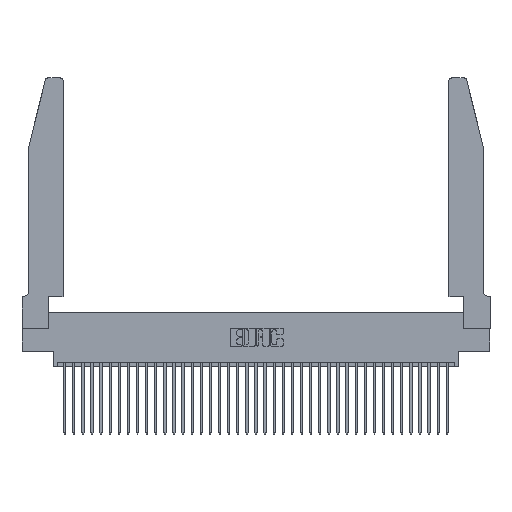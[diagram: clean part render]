
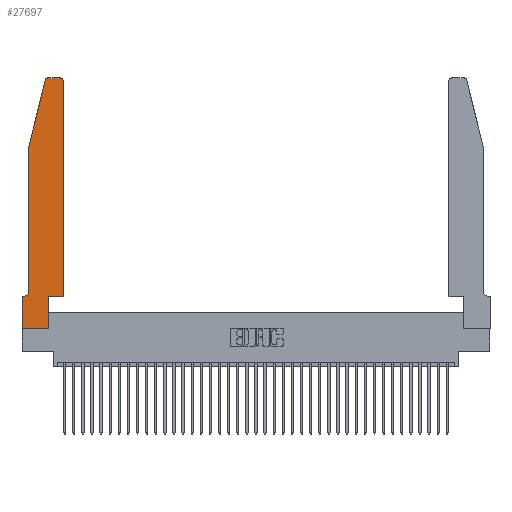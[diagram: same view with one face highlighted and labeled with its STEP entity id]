
A CAD part, top view. The second image highlights one B-rep face of the part: STEP entity #27697.
In plain terms, the highlighted planar face has unit normal (0, 0, 1).
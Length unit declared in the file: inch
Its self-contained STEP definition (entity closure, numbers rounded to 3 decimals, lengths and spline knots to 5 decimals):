
#157 = VECTOR ( 'NONE', #2170, 39.37008 ) ;
#538 = LINE ( 'NONE', #36067, #36843 ) ;
#541 = AXIS2_PLACEMENT_3D ( 'NONE', #23061, #37790, #2032 ) ;
#722 = ORIENTED_EDGE ( 'NONE', *, *, #15746, .T. ) ;
#992 = CARTESIAN_POINT ( 'NONE',  ( 0.2865, 0.35, 0.37 ) ) ;
#1665 = DIRECTION ( 'NONE',  ( -1., 0., 0. ) ) ;
#2032 = DIRECTION ( 'NONE',  ( 1., 0., 0. ) ) ;
#2036 = DIRECTION ( 'NONE',  ( 0., 0., 1. ) ) ;
#2053 = DIRECTION ( 'NONE',  ( 0., 1., 0. ) ) ;
#2170 = DIRECTION ( 'NONE',  ( 0., -1., 0. ) ) ;
#2722 = LINE ( 'NONE', #25819, #16658 ) ;
#2791 = CARTESIAN_POINT ( 'NONE',  ( 0.0755, 2., 0.37 ) ) ;
#3382 = EDGE_CURVE ( 'NONE', #18081, #23666, #15331, .T. ) ;
#3668 = CARTESIAN_POINT ( 'NONE',  ( 0.25487, 2.72718, 0.37 ) ) ;
#3932 = CARTESIAN_POINT ( 'NONE',  ( 0.0755, 0.35, 0.37 ) ) ;
#4237 = VECTOR ( 'NONE', #12167, 39.37008 ) ;
#5111 = EDGE_CURVE ( 'NONE', #26515, #19063, #26829, .T. ) ;
#5222 = VECTOR ( 'NONE', #24670, 39.37008 ) ;
#6539 = CARTESIAN_POINT ( 'NONE',  ( 0.4205, 2.72, 0.37 ) ) ;
#7099 = VERTEX_POINT ( 'NONE', #992 ) ;
#7394 = LINE ( 'NONE', #31576, #28295 ) ;
#7828 = ORIENTED_EDGE ( 'NONE', *, *, #9052, .T. ) ;
#7960 = EDGE_CURVE ( 'NONE', #37429, #7099, #31318, .T. ) ;
#8455 = CARTESIAN_POINT ( 'NONE',  ( 0.284, 2.75, 0.37 ) ) ;
#9052 = EDGE_CURVE ( 'NONE', #32411, #11761, #12148, .T. ) ;
#10139 = CARTESIAN_POINT ( 'NONE',  ( 0.0755, 0.42, 0.37 ) ) ;
#10618 = LINE ( 'NONE', #22981, #24497 ) ;
#10767 = LINE ( 'NONE', #3932, #5222 ) ;
#10826 = CARTESIAN_POINT ( 'NONE',  ( 0.4205, 2.75, 0.37 ) ) ;
#10954 = AXIS2_PLACEMENT_3D ( 'NONE', #37665, #2036, #23834 ) ;
#11626 = ORIENTED_EDGE ( 'NONE', *, *, #17884, .T. ) ;
#11761 = VERTEX_POINT ( 'NONE', #14940 ) ;
#11939 = CARTESIAN_POINT ( 'NONE',  ( 0.2865, 0., 0.37 ) ) ;
#12148 = LINE ( 'NONE', #33376, #4237 ) ;
#12167 = DIRECTION ( 'NONE',  ( 0., -1., 0. ) ) ;
#12203 = AXIS2_PLACEMENT_3D ( 'NONE', #6539, #12526, #32969 ) ;
#12499 = ORIENTED_EDGE ( 'NONE', *, *, #3382, .T. ) ;
#12526 = DIRECTION ( 'NONE',  ( 0., 0., 1. ) ) ;
#12634 = DIRECTION ( 'NONE',  ( -1., 0., 0. ) ) ;
#12736 = EDGE_LOOP ( 'NONE', ( #722, #12499, #11626, #36169, #35015, #14426, #7828, #24237, #23071, #22377, #35785, #23456 ) ) ;
#12743 = CARTESIAN_POINT ( 'NONE',  ( 0.0055, 0.35, 0.37 ) ) ;
#13341 = EDGE_CURVE ( 'NONE', #32040, #32411, #10767, .T. ) ;
#14426 = ORIENTED_EDGE ( 'NONE', *, *, #13341, .T. ) ;
#14827 = EDGE_CURVE ( 'NONE', #36055, #20274, #21537, .T. ) ;
#14940 = CARTESIAN_POINT ( 'NONE',  ( 0., 0., 0.37 ) ) ;
#15030 = CARTESIAN_POINT ( 'NONE',  ( 0., 0.35, 0.37 ) ) ;
#15331 = CIRCLE ( 'NONE', #10954, 0.03 ) ;
#15500 = DIRECTION ( 'NONE',  ( 0., 1., 0. ) ) ;
#15746 = EDGE_CURVE ( 'NONE', #19063, #18081, #538, .T. ) ;
#16603 = DIRECTION ( 'NONE',  ( -0.239, -0.971, 0. ) ) ;
#16658 = VECTOR ( 'NONE', #2053, 39.37008 ) ;
#17102 = CARTESIAN_POINT ( 'NONE',  ( 0.0755, 2., 0.37 ) ) ;
#17884 = EDGE_CURVE ( 'NONE', #23666, #36055, #7394, .T. ) ;
#18081 = VERTEX_POINT ( 'NONE', #8455 ) ;
#18486 = EDGE_CURVE ( 'NONE', #7099, #24589, #33867, .T. ) ;
#18702 = VECTOR ( 'NONE', #15500, 39.37008 ) ;
#19063 = VERTEX_POINT ( 'NONE', #10826 ) ;
#19673 = EDGE_CURVE ( 'NONE', #20274, #32040, #37438, .T. ) ;
#19682 = CARTESIAN_POINT ( 'NONE',  ( 0.4505, 0.35, 0.37 ) ) ;
#20274 = VERTEX_POINT ( 'NONE', #10139 ) ;
#21537 = LINE ( 'NONE', #17102, #157 ) ;
#22377 = ORIENTED_EDGE ( 'NONE', *, *, #18486, .T. ) ;
#22981 = CARTESIAN_POINT ( 'NONE',  ( 0., 0., 0.37 ) ) ;
#23061 = CARTESIAN_POINT ( 'NONE',  ( 0., 0.35, 0.37 ) ) ;
#23071 = ORIENTED_EDGE ( 'NONE', *, *, #7960, .T. ) ;
#23456 = ORIENTED_EDGE ( 'NONE', *, *, #5111, .T. ) ;
#23666 = VERTEX_POINT ( 'NONE', #3668 ) ;
#23834 = DIRECTION ( 'NONE',  ( 1., 0., 0. ) ) ;
#24237 = ORIENTED_EDGE ( 'NONE', *, *, #31456, .T. ) ;
#24497 = VECTOR ( 'NONE', #32136, 39.37008 ) ;
#24589 = VERTEX_POINT ( 'NONE', #19682 ) ;
#24670 = DIRECTION ( 'NONE',  ( -1., 0., 0. ) ) ;
#25037 = CARTESIAN_POINT ( 'NONE',  ( 0.0055, 0.42, 0.37 ) ) ;
#25819 = CARTESIAN_POINT ( 'NONE',  ( 0.4505, 0.35, 0.37 ) ) ;
#26515 = VERTEX_POINT ( 'NONE', #30187 ) ;
#26829 = CIRCLE ( 'NONE', #12203, 0.03 ) ;
#27472 = CARTESIAN_POINT ( 'NONE',  ( 0.2865, 0.35, 0.37 ) ) ;
#27550 = AXIS2_PLACEMENT_3D ( 'NONE', #25037, #37178, #1665 ) ;
#27697 = ADVANCED_FACE ( 'NONE', ( #33197 ), #37663, .T. ) ;
#28295 = VECTOR ( 'NONE', #16603, 39.37008 ) ;
#30176 = EDGE_CURVE ( 'NONE', #24589, #26515, #2722, .T. ) ;
#30187 = CARTESIAN_POINT ( 'NONE',  ( 0.4505, 2.72, 0.37 ) ) ;
#30617 = DIRECTION ( 'NONE',  ( 1., 0., 0. ) ) ;
#31318 = LINE ( 'NONE', #27472, #18702 ) ;
#31456 = EDGE_CURVE ( 'NONE', #11761, #37429, #10618, .T. ) ;
#31576 = CARTESIAN_POINT ( 'NONE',  ( 0.0755, 2., 0.37 ) ) ;
#32040 = VERTEX_POINT ( 'NONE', #12743 ) ;
#32136 = DIRECTION ( 'NONE',  ( 1., 0., 0. ) ) ;
#32411 = VERTEX_POINT ( 'NONE', #15030 ) ;
#32969 = DIRECTION ( 'NONE',  ( 1., 0., 0. ) ) ;
#33197 = FACE_OUTER_BOUND ( 'NONE', #12736, .T. ) ;
#33376 = CARTESIAN_POINT ( 'NONE',  ( 0., 0., 0.37 ) ) ;
#33797 = CARTESIAN_POINT ( 'NONE',  ( 0.4505, 0.35, 0.37 ) ) ;
#33867 = LINE ( 'NONE', #33797, #37554 ) ;
#35015 = ORIENTED_EDGE ( 'NONE', *, *, #19673, .T. ) ;
#35785 = ORIENTED_EDGE ( 'NONE', *, *, #30176, .T. ) ;
#36055 = VERTEX_POINT ( 'NONE', #2791 ) ;
#36067 = CARTESIAN_POINT ( 'NONE',  ( 0.2605, 2.75, 0.37 ) ) ;
#36169 = ORIENTED_EDGE ( 'NONE', *, *, #14827, .T. ) ;
#36843 = VECTOR ( 'NONE', #12634, 39.37008 ) ;
#37178 = DIRECTION ( 'NONE',  ( 0., 0., -1. ) ) ;
#37429 = VERTEX_POINT ( 'NONE', #11939 ) ;
#37438 = CIRCLE ( 'NONE', #27550, 0.07 ) ;
#37554 = VECTOR ( 'NONE', #30617, 39.37008 ) ;
#37663 = PLANE ( 'NONE',  #541 ) ;
#37665 = CARTESIAN_POINT ( 'NONE',  ( 0.284, 2.72, 0.37 ) ) ;
#37790 = DIRECTION ( 'NONE',  ( 0., 0., 1. ) ) ;
